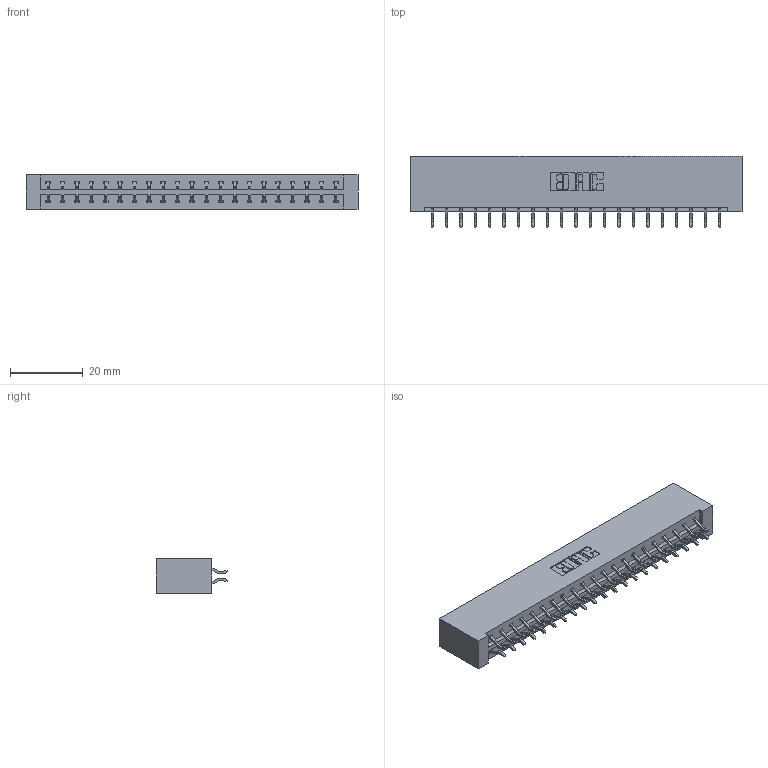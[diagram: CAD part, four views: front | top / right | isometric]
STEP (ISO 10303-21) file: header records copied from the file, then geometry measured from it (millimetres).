
FILE_DESCRIPTION (( 'STEP AP203' ), '1' );
FILE_NAME ('333-042-556-201.STEP', '2018-08-03T19:27:29', ( '' ), ( '' ), 'SwSTEP 2.0', 'SolidWorks 2016', '' );
FILE_SCHEMA (( 'CONFIG_CONTROL_DESIGN' ));
Length unit declared in the file: inch
Products named in the file (3): 333 Part_Lugless; 345-292-001_556 Tail; 333-042-556-201
Assembly tree (43 placements, depth 2):
  333-042-556-201
    333 Part_Lugless
    345-292-001_556 Tail  x42
Bounding box: 91.47 x 19.57 x 9.4 mm (x, y, z)
Volume: 9772.3 mm3; surface area: 11310.5 mm2
Topology: 43 solids, 43 shells, 2542 faces, 7553 edges, 4978 vertices
Faces by surface type: plane 1746, cylinder 796
Entity records: 16169 total; most frequent: CARTESIAN_POINT 2718, ORIENTED_EDGE 2642, DIRECTION 2341, EDGE_CURVE 1321, VECTOR 1193, LINE 1193, VERTEX_POINT 878, AXIS2_PLACEMENT_3D 574
